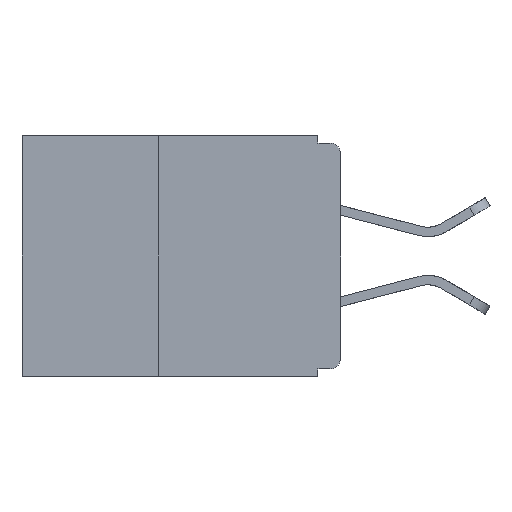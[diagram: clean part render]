
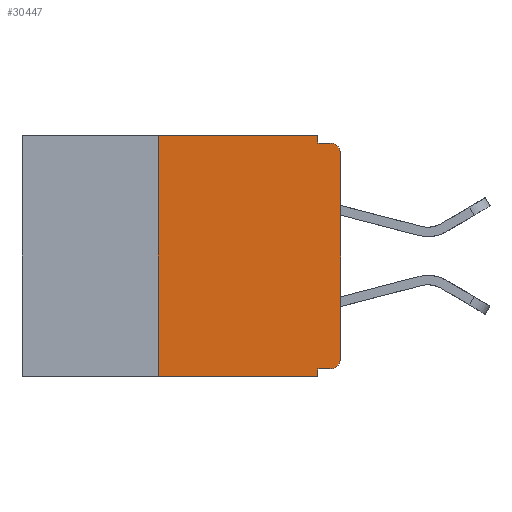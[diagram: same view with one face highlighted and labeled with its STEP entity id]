
A CAD part, left-side view. The second image highlights one B-rep face of the part: STEP entity #30447.
In plain terms, the highlighted planar face has unit normal (-1, 0, 0).
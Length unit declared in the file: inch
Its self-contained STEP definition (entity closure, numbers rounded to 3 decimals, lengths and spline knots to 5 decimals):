
#128 = DIRECTION ( 'NONE',  ( 0., -1., 0. ) ) ;
#878 = CARTESIAN_POINT ( 'NONE',  ( 0., 0.015, -0.01 ) ) ;
#1218 = DIRECTION ( 'NONE',  ( 0., 1., 0. ) ) ;
#1494 = ORIENTED_EDGE ( 'NONE', *, *, #24638, .F. ) ;
#1754 = DIRECTION ( 'NONE',  ( 0., 0., -1. ) ) ;
#1935 = CARTESIAN_POINT ( 'NONE',  ( 0., 0.25, 0. ) ) ;
#2132 = CARTESIAN_POINT ( 'NONE',  ( 0., 0.015, -0.32 ) ) ;
#2394 = DIRECTION ( 'NONE',  ( 1., 0., 0. ) ) ;
#3266 = CARTESIAN_POINT ( 'NONE',  ( 0., 0.25, -0.33 ) ) ;
#4935 = DIRECTION ( 'NONE',  ( 0., 0., 1. ) ) ;
#4940 = DIRECTION ( 'NONE',  ( 0., 0., -1. ) ) ;
#5092 = VERTEX_POINT ( 'NONE', #12221 ) ;
#5927 = EDGE_CURVE ( 'NONE', #9365, #23077, #28797, .T. ) ;
#5958 = VERTEX_POINT ( 'NONE', #27867 ) ;
#6310 = ORIENTED_EDGE ( 'NONE', *, *, #18720, .F. ) ;
#6806 = VECTOR ( 'NONE', #128, 39.37008 ) ;
#6991 = EDGE_CURVE ( 'NONE', #35399, #5958, #24427, .T. ) ;
#7315 = VERTEX_POINT ( 'NONE', #8712 ) ;
#7392 = EDGE_CURVE ( 'NONE', #7315, #24401, #25247, .T. ) ;
#8712 = CARTESIAN_POINT ( 'NONE',  ( 0., 0., -0.025 ) ) ;
#9073 = EDGE_CURVE ( 'NONE', #5958, #7315, #31325, .T. ) ;
#9365 = VERTEX_POINT ( 'NONE', #3266 ) ;
#9442 = ORIENTED_EDGE ( 'NONE', *, *, #7392, .T. ) ;
#10091 = ORIENTED_EDGE ( 'NONE', *, *, #24209, .T. ) ;
#10485 = CARTESIAN_POINT ( 'NONE',  ( 0., 0., 0. ) ) ;
#11657 = LINE ( 'NONE', #20517, #20093 ) ;
#12221 = CARTESIAN_POINT ( 'NONE',  ( 0., 0.031, -0.33 ) ) ;
#12345 = CARTESIAN_POINT ( 'NONE',  ( 0., 0.015, -0.025 ) ) ;
#12535 = ORIENTED_EDGE ( 'NONE', *, *, #32297, .F. ) ;
#13277 = CARTESIAN_POINT ( 'NONE',  ( 0., 0.031, 0. ) ) ;
#13628 = VERTEX_POINT ( 'NONE', #26778 ) ;
#15084 = CARTESIAN_POINT ( 'NONE',  ( 0., 0.031, -0.33 ) ) ;
#15173 = ORIENTED_EDGE ( 'NONE', *, *, #6991, .T. ) ;
#15178 = LINE ( 'NONE', #28308, #6806 ) ;
#15205 = DIRECTION ( 'NONE',  ( 0., 0., -1. ) ) ;
#16344 = DIRECTION ( 'NONE',  ( 0., -1., 0. ) ) ;
#16575 = VECTOR ( 'NONE', #4940, 39.37008 ) ;
#17447 = LINE ( 'NONE', #13277, #16575 ) ;
#17646 = LINE ( 'NONE', #15084, #25153 ) ;
#18720 = EDGE_CURVE ( 'NONE', #35399, #19305, #31977, .T. ) ;
#18741 = DIRECTION ( 'NONE',  ( -1., 0., 0. ) ) ;
#19305 = VERTEX_POINT ( 'NONE', #20894 ) ;
#20093 = VECTOR ( 'NONE', #31662, 39.37008 ) ;
#20469 = ORIENTED_EDGE ( 'NONE', *, *, #32582, .F. ) ;
#20509 = VECTOR ( 'NONE', #27746, 39.37008 ) ;
#20517 = CARTESIAN_POINT ( 'NONE',  ( 0., 0.437, 0. ) ) ;
#20894 = CARTESIAN_POINT ( 'NONE',  ( 0., 0.031, -0.32 ) ) ;
#21741 = VERTEX_POINT ( 'NONE', #34706 ) ;
#22073 = CARTESIAN_POINT ( 'NONE',  ( 0., 0.437, 0. ) ) ;
#22184 = DIRECTION ( 'NONE',  ( 0., 0., -1. ) ) ;
#22222 = FACE_OUTER_BOUND ( 'NONE', #25825, .T. ) ;
#23077 = VERTEX_POINT ( 'NONE', #1935 ) ;
#23797 = LINE ( 'NONE', #30258, #30284 ) ;
#24011 = VECTOR ( 'NONE', #4935, 39.37008 ) ;
#24209 = EDGE_CURVE ( 'NONE', #9365, #5092, #15178, .T. ) ;
#24401 = VERTEX_POINT ( 'NONE', #878 ) ;
#24427 = CIRCLE ( 'NONE', #29868, 0.015 ) ;
#24638 = EDGE_CURVE ( 'NONE', #21741, #13628, #17447, .T. ) ;
#25153 = VECTOR ( 'NONE', #29065, 39.37008 ) ;
#25247 = CIRCLE ( 'NONE', #34679, 0.015 ) ;
#25825 = EDGE_LOOP ( 'NONE', ( #36153, #9442, #20469, #1494, #33260, #28534, #10091, #12535, #6310, #15173 ) ) ;
#26778 = CARTESIAN_POINT ( 'NONE',  ( 0., 0.031, -0.01 ) ) ;
#27746 = DIRECTION ( 'NONE',  ( 0., 0., 1. ) ) ;
#27867 = CARTESIAN_POINT ( 'NONE',  ( 0., 0., -0.305 ) ) ;
#28308 = CARTESIAN_POINT ( 'NONE',  ( 0., 0.437, -0.33 ) ) ;
#28534 = ORIENTED_EDGE ( 'NONE', *, *, #5927, .F. ) ;
#28797 = LINE ( 'NONE', #35845, #20509 ) ;
#29065 = DIRECTION ( 'NONE',  ( 0., 0., -1. ) ) ;
#29323 = CARTESIAN_POINT ( 'NONE',  ( 0., 0., -0.32 ) ) ;
#29464 = EDGE_CURVE ( 'NONE', #23077, #21741, #11657, .T. ) ;
#29868 = AXIS2_PLACEMENT_3D ( 'NONE', #35280, #18741, #1754 ) ;
#30258 = CARTESIAN_POINT ( 'NONE',  ( 0., 0., -0.01 ) ) ;
#30284 = VECTOR ( 'NONE', #16344, 39.37008 ) ;
#30447 = ADVANCED_FACE ( 'NONE', ( #22222 ), #35897, .F. ) ;
#30633 = AXIS2_PLACEMENT_3D ( 'NONE', #22073, #2394, #22184 ) ;
#31123 = VECTOR ( 'NONE', #1218, 39.37008 ) ;
#31325 = LINE ( 'NONE', #10485, #24011 ) ;
#31662 = DIRECTION ( 'NONE',  ( 0., -1., 0. ) ) ;
#31937 = DIRECTION ( 'NONE',  ( -1., 0., 0. ) ) ;
#31977 = LINE ( 'NONE', #29323, #31123 ) ;
#32297 = EDGE_CURVE ( 'NONE', #19305, #5092, #17646, .T. ) ;
#32582 = EDGE_CURVE ( 'NONE', #13628, #24401, #23797, .T. ) ;
#33260 = ORIENTED_EDGE ( 'NONE', *, *, #29464, .F. ) ;
#34679 = AXIS2_PLACEMENT_3D ( 'NONE', #12345, #31937, #15205 ) ;
#34706 = CARTESIAN_POINT ( 'NONE',  ( 0., 0.031, 0. ) ) ;
#35280 = CARTESIAN_POINT ( 'NONE',  ( 0., 0.015, -0.305 ) ) ;
#35399 = VERTEX_POINT ( 'NONE', #2132 ) ;
#35845 = CARTESIAN_POINT ( 'NONE',  ( 0., 0.25, -0.33 ) ) ;
#35897 = PLANE ( 'NONE',  #30633 ) ;
#36153 = ORIENTED_EDGE ( 'NONE', *, *, #9073, .T. ) ;
